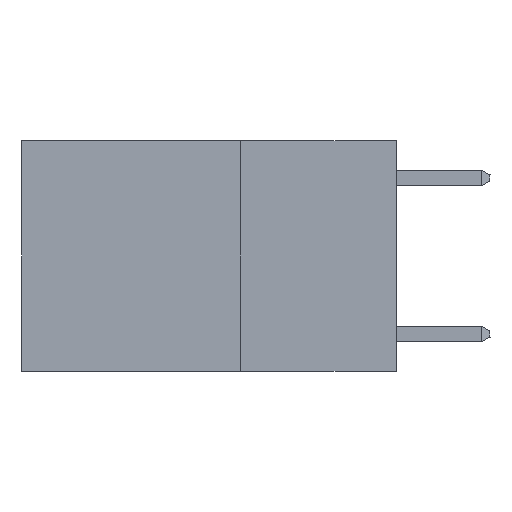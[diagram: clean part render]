
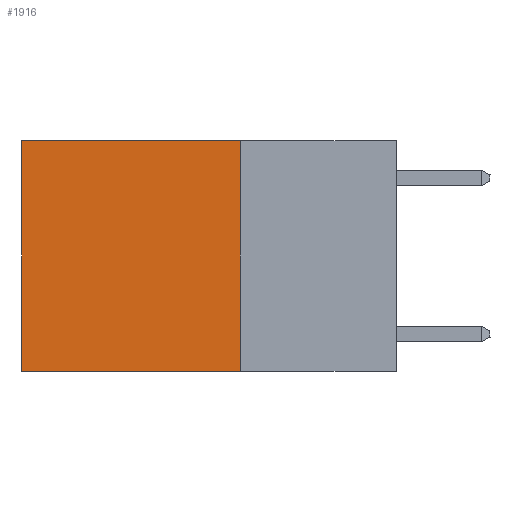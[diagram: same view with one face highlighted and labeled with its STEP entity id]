
A CAD part, left-side view. The second image highlights one B-rep face of the part: STEP entity #1916.
In plain terms, the highlighted planar face has unit normal (-1, 0, 0).
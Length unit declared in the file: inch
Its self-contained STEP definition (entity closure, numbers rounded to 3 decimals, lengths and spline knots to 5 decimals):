
#217 = LINE ( 'NONE', #5809, #9334 ) ;
#1205 = EDGE_CURVE ( 'NONE', #11546, #1895, #6048, .T. ) ;
#1355 = CARTESIAN_POINT ( 'NONE',  ( 0.2625, 0.25, 0. ) ) ;
#1895 = VERTEX_POINT ( 'NONE', #9280 ) ;
#1916 = ADVANCED_FACE ( 'NONE', ( #2018 ), #2870, .F. ) ;
#2018 = FACE_OUTER_BOUND ( 'NONE', #5785, .T. ) ;
#2049 = DIRECTION ( 'NONE',  ( 0., 1., 0. ) ) ;
#2224 = CARTESIAN_POINT ( 'NONE',  ( 0.2625, 0.25, 0. ) ) ;
#2315 = VECTOR ( 'NONE', #9913, 39.37008 ) ;
#2466 = ORIENTED_EDGE ( 'NONE', *, *, #4143, .T. ) ;
#2680 = DIRECTION ( 'NONE',  ( 1., 0., 0. ) ) ;
#2870 = PLANE ( 'NONE',  #4906 ) ;
#2975 = DIRECTION ( 'NONE',  ( 0., 1., 0. ) ) ;
#2995 = EDGE_CURVE ( 'NONE', #11546, #7016, #10388, .T. ) ;
#3013 = VECTOR ( 'NONE', #2049, 39.37008 ) ;
#3203 = DIRECTION ( 'NONE',  ( 0., 0., -1. ) ) ;
#3335 = LINE ( 'NONE', #8044, #2315 ) ;
#3603 = DIRECTION ( 'NONE',  ( 0., 0., -1. ) ) ;
#4143 = EDGE_CURVE ( 'NONE', #7016, #12003, #3335, .T. ) ;
#4826 = ORIENTED_EDGE ( 'NONE', *, *, #7730, .F. ) ;
#4906 = AXIS2_PLACEMENT_3D ( 'NONE', #6344, #2680, #3603 ) ;
#5785 = EDGE_LOOP ( 'NONE', ( #2466, #4826, #6122, #10060 ) ) ;
#5809 = CARTESIAN_POINT ( 'NONE',  ( 0.2625, 0.25, -0.37 ) ) ;
#5857 = CARTESIAN_POINT ( 'NONE',  ( 0.2625, 0.6, 0. ) ) ;
#6048 = LINE ( 'NONE', #2224, #9002 ) ;
#6122 = ORIENTED_EDGE ( 'NONE', *, *, #1205, .F. ) ;
#6344 = CARTESIAN_POINT ( 'NONE',  ( 0.2625, 0.25, 0. ) ) ;
#7016 = VERTEX_POINT ( 'NONE', #5857 ) ;
#7730 = EDGE_CURVE ( 'NONE', #1895, #12003, #217, .T. ) ;
#7970 = CARTESIAN_POINT ( 'NONE',  ( 0.2625, 0.6, -0.37 ) ) ;
#8044 = CARTESIAN_POINT ( 'NONE',  ( 0.2625, 0.6, 0. ) ) ;
#9002 = VECTOR ( 'NONE', #3203, 39.37008 ) ;
#9280 = CARTESIAN_POINT ( 'NONE',  ( 0.2625, 0.25, -0.37 ) ) ;
#9334 = VECTOR ( 'NONE', #2975, 39.37008 ) ;
#9913 = DIRECTION ( 'NONE',  ( 0., 0., -1. ) ) ;
#10060 = ORIENTED_EDGE ( 'NONE', *, *, #2995, .T. ) ;
#10388 = LINE ( 'NONE', #11252, #3013 ) ;
#11252 = CARTESIAN_POINT ( 'NONE',  ( 0.2625, 0.25, 0. ) ) ;
#11546 = VERTEX_POINT ( 'NONE', #1355 ) ;
#12003 = VERTEX_POINT ( 'NONE', #7970 ) ;
